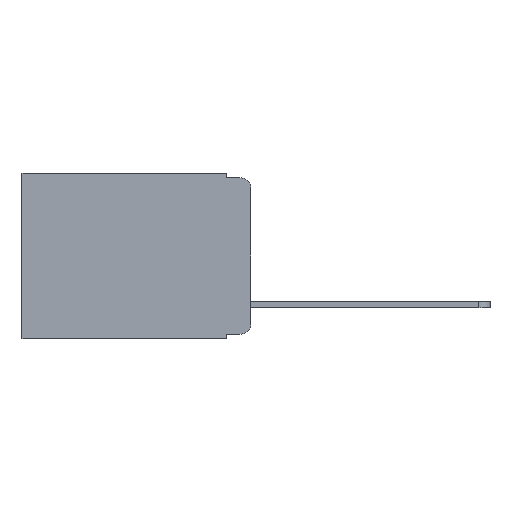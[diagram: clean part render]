
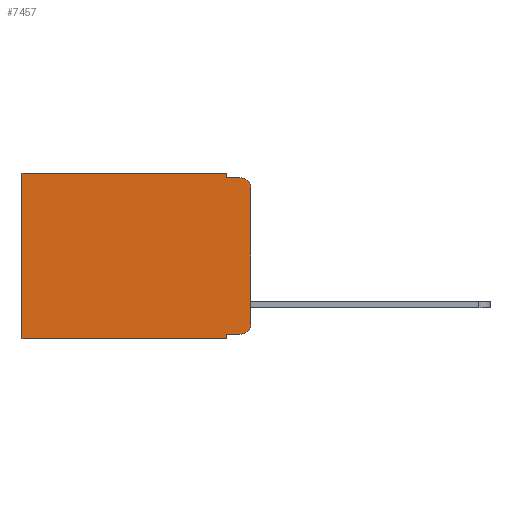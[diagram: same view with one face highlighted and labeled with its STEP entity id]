
A CAD part, left-side view. The second image highlights one B-rep face of the part: STEP entity #7457.
In plain terms, the highlighted planar face has unit normal (-1, 0, 0).
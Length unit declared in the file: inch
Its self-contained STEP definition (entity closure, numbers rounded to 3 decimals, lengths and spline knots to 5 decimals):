
#162 = VECTOR ( 'NONE', #13425, 39.37008 ) ;
#227 = ORIENTED_EDGE ( 'NONE', *, *, #9490, .T. ) ;
#498 = VECTOR ( 'NONE', #13364, 39.37008 ) ;
#544 = CARTESIAN_POINT ( 'NONE',  ( 0.298, 0.02, -0.313 ) ) ;
#1050 = CARTESIAN_POINT ( 'NONE',  ( 0.298, 0., -0.343 ) ) ;
#1290 = VECTOR ( 'NONE', #3305, 39.37008 ) ;
#1303 = ORIENTED_EDGE ( 'NONE', *, *, #5419, .F. ) ;
#1379 = VERTEX_POINT ( 'NONE', #8870 ) ;
#1477 = DIRECTION ( 'NONE',  ( 0., 0., -1. ) ) ;
#2312 = CARTESIAN_POINT ( 'NONE',  ( 0.298, 0., 0. ) ) ;
#2463 = FACE_OUTER_BOUND ( 'NONE', #5914, .T. ) ;
#2510 = AXIS2_PLACEMENT_3D ( 'NONE', #544, #6043, #13835 ) ;
#2511 = CARTESIAN_POINT ( 'NONE',  ( 0.298, 0.051, -0.333 ) ) ;
#2517 = DIRECTION ( 'NONE',  ( 0., 0., -1. ) ) ;
#2590 = VERTEX_POINT ( 'NONE', #4707 ) ;
#3021 = VECTOR ( 'NONE', #2517, 39.37008 ) ;
#3023 = CARTESIAN_POINT ( 'NONE',  ( 0.298, 0., -0.313 ) ) ;
#3305 = DIRECTION ( 'NONE',  ( 0., 0., -1. ) ) ;
#3431 = LINE ( 'NONE', #7899, #4854 ) ;
#3462 = LINE ( 'NONE', #1050, #11371 ) ;
#3526 = DIRECTION ( 'NONE',  ( 0., -1., 0. ) ) ;
#3747 = CARTESIAN_POINT ( 'NONE',  ( 0.298, 0.473, -0.343 ) ) ;
#3769 = CARTESIAN_POINT ( 'NONE',  ( 0.298, 0., 0. ) ) ;
#4483 = LINE ( 'NONE', #12135, #1290 ) ;
#4638 = CARTESIAN_POINT ( 'NONE',  ( 0.298, 0.051, 0. ) ) ;
#4707 = CARTESIAN_POINT ( 'NONE',  ( 0.298, 0.473, 0. ) ) ;
#4802 = VECTOR ( 'NONE', #13976, 39.37008 ) ;
#4817 = EDGE_CURVE ( 'NONE', #13897, #12284, #8332, .T. ) ;
#4854 = VECTOR ( 'NONE', #12262, 39.37008 ) ;
#5030 = EDGE_CURVE ( 'NONE', #10529, #8294, #3462, .T. ) ;
#5071 = CARTESIAN_POINT ( 'NONE',  ( 0.298, 0., -0.03 ) ) ;
#5208 = VERTEX_POINT ( 'NONE', #12921 ) ;
#5419 = EDGE_CURVE ( 'NONE', #10923, #12284, #8985, .T. ) ;
#5463 = AXIS2_PLACEMENT_3D ( 'NONE', #2312, #13467, #12449 ) ;
#5797 = CARTESIAN_POINT ( 'NONE',  ( 0.298, 0.051, -0.01 ) ) ;
#5914 = EDGE_LOOP ( 'NONE', ( #1303, #12119, #10880, #10474, #7688, #227, #10353, #8086, #14264, #6106 ) ) ;
#6034 = VERTEX_POINT ( 'NONE', #6476 ) ;
#6043 = DIRECTION ( 'NONE',  ( -1., 0., 0. ) ) ;
#6106 = ORIENTED_EDGE ( 'NONE', *, *, #4817, .T. ) ;
#6476 = CARTESIAN_POINT ( 'NONE',  ( 0.298, 0.051, -0.333 ) ) ;
#6659 = LINE ( 'NONE', #5797, #498 ) ;
#7186 = DIRECTION ( 'NONE',  ( -1., 0., 0. ) ) ;
#7457 = ADVANCED_FACE ( 'NONE', ( #2463 ), #8005, .F. ) ;
#7688 = ORIENTED_EDGE ( 'NONE', *, *, #9163, .T. ) ;
#7856 = DIRECTION ( 'NONE',  ( 0., 1., 0. ) ) ;
#7899 = CARTESIAN_POINT ( 'NONE',  ( 0.298, 0.051, 0. ) ) ;
#7983 = CARTESIAN_POINT ( 'NONE',  ( 0.298, 0.051, -0.01 ) ) ;
#8005 = PLANE ( 'NONE',  #5463 ) ;
#8086 = ORIENTED_EDGE ( 'NONE', *, *, #12403, .F. ) ;
#8177 = CARTESIAN_POINT ( 'NONE',  ( 0.298, 0., 0. ) ) ;
#8202 = VERTEX_POINT ( 'NONE', #7983 ) ;
#8294 = VERTEX_POINT ( 'NONE', #3747 ) ;
#8332 = CIRCLE ( 'NONE', #2510, 0.02 ) ;
#8870 = CARTESIAN_POINT ( 'NONE',  ( 0.298, 0.051, 0. ) ) ;
#8985 = LINE ( 'NONE', #8177, #162 ) ;
#9163 = EDGE_CURVE ( 'NONE', #1379, #2590, #13903, .T. ) ;
#9490 = EDGE_CURVE ( 'NONE', #2590, #8294, #4483, .T. ) ;
#9605 = EDGE_CURVE ( 'NONE', #10923, #5208, #13417, .T. ) ;
#10353 = ORIENTED_EDGE ( 'NONE', *, *, #5030, .F. ) ;
#10474 = ORIENTED_EDGE ( 'NONE', *, *, #11240, .F. ) ;
#10529 = VERTEX_POINT ( 'NONE', #11789 ) ;
#10701 = EDGE_CURVE ( 'NONE', #6034, #13897, #13522, .T. ) ;
#10880 = ORIENTED_EDGE ( 'NONE', *, *, #14029, .F. ) ;
#10923 = VERTEX_POINT ( 'NONE', #5071 ) ;
#11240 = EDGE_CURVE ( 'NONE', #1379, #8202, #3431, .T. ) ;
#11371 = VECTOR ( 'NONE', #7856, 39.37008 ) ;
#11789 = CARTESIAN_POINT ( 'NONE',  ( 0.298, 0.051, -0.343 ) ) ;
#11803 = VECTOR ( 'NONE', #3526, 39.37008 ) ;
#12013 = AXIS2_PLACEMENT_3D ( 'NONE', #12648, #7186, #1477 ) ;
#12053 = CARTESIAN_POINT ( 'NONE',  ( 0.298, 0.02, -0.333 ) ) ;
#12119 = ORIENTED_EDGE ( 'NONE', *, *, #9605, .T. ) ;
#12135 = CARTESIAN_POINT ( 'NONE',  ( 0.298, 0.473, 0. ) ) ;
#12262 = DIRECTION ( 'NONE',  ( 0., 0., -1. ) ) ;
#12284 = VERTEX_POINT ( 'NONE', #3023 ) ;
#12403 = EDGE_CURVE ( 'NONE', #6034, #10529, #13603, .T. ) ;
#12449 = DIRECTION ( 'NONE',  ( 0., 0., -1. ) ) ;
#12648 = CARTESIAN_POINT ( 'NONE',  ( 0.298, 0.02, -0.03 ) ) ;
#12921 = CARTESIAN_POINT ( 'NONE',  ( 0.298, 0.02, -0.01 ) ) ;
#13364 = DIRECTION ( 'NONE',  ( 0., -1., 0. ) ) ;
#13417 = CIRCLE ( 'NONE', #12013, 0.02 ) ;
#13425 = DIRECTION ( 'NONE',  ( 0., 0., -1. ) ) ;
#13467 = DIRECTION ( 'NONE',  ( 1., 0., 0. ) ) ;
#13522 = LINE ( 'NONE', #2511, #11803 ) ;
#13603 = LINE ( 'NONE', #4638, #3021 ) ;
#13835 = DIRECTION ( 'NONE',  ( 0., 0., -1. ) ) ;
#13897 = VERTEX_POINT ( 'NONE', #12053 ) ;
#13903 = LINE ( 'NONE', #3769, #4802 ) ;
#13976 = DIRECTION ( 'NONE',  ( 0., 1., 0. ) ) ;
#14029 = EDGE_CURVE ( 'NONE', #8202, #5208, #6659, .T. ) ;
#14264 = ORIENTED_EDGE ( 'NONE', *, *, #10701, .T. ) ;
